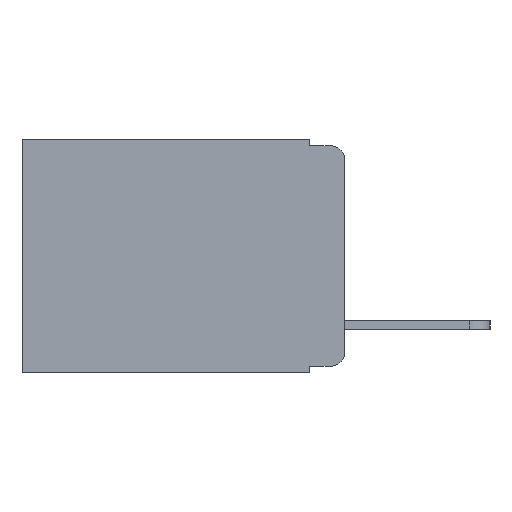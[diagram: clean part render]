
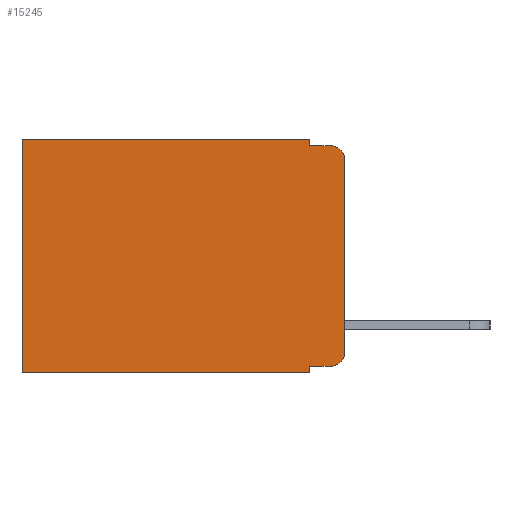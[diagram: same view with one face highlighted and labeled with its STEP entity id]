
A CAD part, left-side view. The second image highlights one B-rep face of the part: STEP entity #15245.
In plain terms, the highlighted planar face has unit normal (-1, 0, 0).
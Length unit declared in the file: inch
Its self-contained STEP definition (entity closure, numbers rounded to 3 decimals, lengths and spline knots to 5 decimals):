
#804 = EDGE_CURVE ( 'NONE', #1659, #19259, #18995, .T. ) ;
#1427 = ORIENTED_EDGE ( 'NONE', *, *, #19930, .F. ) ;
#1541 = VERTEX_POINT ( 'NONE', #19430 ) ;
#1659 = VERTEX_POINT ( 'NONE', #11675 ) ;
#1983 = CARTESIAN_POINT ( 'NONE',  ( 0.298, 0., 0. ) ) ;
#2524 = DIRECTION ( 'NONE',  ( 1., 0., 0. ) ) ;
#2608 = VERTEX_POINT ( 'NONE', #17991 ) ;
#2651 = CARTESIAN_POINT ( 'NONE',  ( 0.298, 0.051, 0. ) ) ;
#3153 = VECTOR ( 'NONE', #8821, 39.37008 ) ;
#3342 = CARTESIAN_POINT ( 'NONE',  ( 0.298, 0.02, -0.03 ) ) ;
#3826 = LINE ( 'NONE', #1983, #6057 ) ;
#3837 = EDGE_LOOP ( 'NONE', ( #9085, #19552, #1427, #15237, #8240, #5613, #4103, #15932, #8895, #5315 ) ) ;
#3910 = EDGE_CURVE ( 'NONE', #18006, #1541, #3826, .T. ) ;
#4018 = VECTOR ( 'NONE', #17475, 39.37008 ) ;
#4103 = ORIENTED_EDGE ( 'NONE', *, *, #4370, .F. ) ;
#4201 = CARTESIAN_POINT ( 'NONE',  ( 0.298, 0.051, -0.333 ) ) ;
#4370 = EDGE_CURVE ( 'NONE', #8781, #20266, #4788, .T. ) ;
#4447 = CARTESIAN_POINT ( 'NONE',  ( 0.298, 0.02, -0.333 ) ) ;
#4701 = FACE_OUTER_BOUND ( 'NONE', #3837, .T. ) ;
#4788 = LINE ( 'NONE', #6445, #17816 ) ;
#5025 = CARTESIAN_POINT ( 'NONE',  ( 0.298, 0.051, 0. ) ) ;
#5315 = ORIENTED_EDGE ( 'NONE', *, *, #8190, .T. ) ;
#5613 = ORIENTED_EDGE ( 'NONE', *, *, #15004, .T. ) ;
#5956 = VECTOR ( 'NONE', #14462, 39.37008 ) ;
#6057 = VECTOR ( 'NONE', #9765, 39.37008 ) ;
#6445 = CARTESIAN_POINT ( 'NONE',  ( 0.298, 0., -0.343 ) ) ;
#6556 = EDGE_CURVE ( 'NONE', #2608, #8781, #13893, .T. ) ;
#6923 = VECTOR ( 'NONE', #17191, 39.37008 ) ;
#7370 = CARTESIAN_POINT ( 'NONE',  ( 0.298, 0.051, -0.01 ) ) ;
#7547 = VERTEX_POINT ( 'NONE', #9221 ) ;
#7624 = DIRECTION ( 'NONE',  ( -1., 0., 0. ) ) ;
#7832 = LINE ( 'NONE', #4201, #3153 ) ;
#7934 = CARTESIAN_POINT ( 'NONE',  ( 0.298, 0.051, -0.01 ) ) ;
#8190 = EDGE_CURVE ( 'NONE', #15485, #1541, #9216, .T. ) ;
#8240 = ORIENTED_EDGE ( 'NONE', *, *, #804, .T. ) ;
#8648 = PLANE ( 'NONE',  #8664 ) ;
#8664 = AXIS2_PLACEMENT_3D ( 'NONE', #11965, #2524, #16770 ) ;
#8781 = VERTEX_POINT ( 'NONE', #13711 ) ;
#8821 = DIRECTION ( 'NONE',  ( 0., -1., 0. ) ) ;
#8895 = ORIENTED_EDGE ( 'NONE', *, *, #17931, .T. ) ;
#8991 = DIRECTION ( 'NONE',  ( 0., 0., -1. ) ) ;
#9085 = ORIENTED_EDGE ( 'NONE', *, *, #3910, .F. ) ;
#9190 = AXIS2_PLACEMENT_3D ( 'NONE', #3342, #14556, #13048 ) ;
#9216 = CIRCLE ( 'NONE', #16793, 0.02 ) ;
#9221 = CARTESIAN_POINT ( 'NONE',  ( 0.298, 0.02, -0.01 ) ) ;
#9341 = DIRECTION ( 'NONE',  ( 0., -1., 0. ) ) ;
#9765 = DIRECTION ( 'NONE',  ( 0., 0., -1. ) ) ;
#9852 = VECTOR ( 'NONE', #8991, 39.37008 ) ;
#10584 = EDGE_CURVE ( 'NONE', #1659, #13709, #18211, .T. ) ;
#10922 = DIRECTION ( 'NONE',  ( 0., 1., 0. ) ) ;
#11094 = VECTOR ( 'NONE', #9341, 39.37008 ) ;
#11675 = CARTESIAN_POINT ( 'NONE',  ( 0.298, 0.051, 0. ) ) ;
#11965 = CARTESIAN_POINT ( 'NONE',  ( 0.298, 0., 0. ) ) ;
#13048 = DIRECTION ( 'NONE',  ( 0., 0., -1. ) ) ;
#13709 = VERTEX_POINT ( 'NONE', #7370 ) ;
#13711 = CARTESIAN_POINT ( 'NONE',  ( 0.298, 0.051, -0.343 ) ) ;
#13893 = LINE ( 'NONE', #5025, #4018 ) ;
#14462 = DIRECTION ( 'NONE',  ( 0., 1., 0. ) ) ;
#14556 = DIRECTION ( 'NONE',  ( -1., 0., 0. ) ) ;
#14774 = LINE ( 'NONE', #7934, #11094 ) ;
#15004 = EDGE_CURVE ( 'NONE', #19259, #20266, #19237, .T. ) ;
#15237 = ORIENTED_EDGE ( 'NONE', *, *, #10584, .F. ) ;
#15245 = ADVANCED_FACE ( 'NONE', ( #4701 ), #8648, .F. ) ;
#15270 = CIRCLE ( 'NONE', #9190, 0.02 ) ;
#15485 = VERTEX_POINT ( 'NONE', #4447 ) ;
#15557 = CARTESIAN_POINT ( 'NONE',  ( 0.298, 0., 0. ) ) ;
#15601 = CARTESIAN_POINT ( 'NONE',  ( 0.298, 0.473, 0. ) ) ;
#15655 = DIRECTION ( 'NONE',  ( 0., 0., -1. ) ) ;
#15704 = EDGE_CURVE ( 'NONE', #18006, #7547, #15270, .T. ) ;
#15932 = ORIENTED_EDGE ( 'NONE', *, *, #6556, .F. ) ;
#16770 = DIRECTION ( 'NONE',  ( 0., 0., -1. ) ) ;
#16793 = AXIS2_PLACEMENT_3D ( 'NONE', #17094, #7624, #15655 ) ;
#17094 = CARTESIAN_POINT ( 'NONE',  ( 0.298, 0.02, -0.313 ) ) ;
#17191 = DIRECTION ( 'NONE',  ( 0., 0., -1. ) ) ;
#17245 = CARTESIAN_POINT ( 'NONE',  ( 0.298, 0.473, 0. ) ) ;
#17475 = DIRECTION ( 'NONE',  ( 0., 0., -1. ) ) ;
#17816 = VECTOR ( 'NONE', #10922, 39.37008 ) ;
#17931 = EDGE_CURVE ( 'NONE', #2608, #15485, #7832, .T. ) ;
#17991 = CARTESIAN_POINT ( 'NONE',  ( 0.298, 0.051, -0.333 ) ) ;
#18006 = VERTEX_POINT ( 'NONE', #18304 ) ;
#18086 = CARTESIAN_POINT ( 'NONE',  ( 0.298, 0.473, -0.343 ) ) ;
#18211 = LINE ( 'NONE', #2651, #9852 ) ;
#18304 = CARTESIAN_POINT ( 'NONE',  ( 0.298, 0., -0.03 ) ) ;
#18995 = LINE ( 'NONE', #15557, #5956 ) ;
#19237 = LINE ( 'NONE', #15601, #6923 ) ;
#19259 = VERTEX_POINT ( 'NONE', #17245 ) ;
#19430 = CARTESIAN_POINT ( 'NONE',  ( 0.298, 0., -0.313 ) ) ;
#19552 = ORIENTED_EDGE ( 'NONE', *, *, #15704, .T. ) ;
#19930 = EDGE_CURVE ( 'NONE', #13709, #7547, #14774, .T. ) ;
#20266 = VERTEX_POINT ( 'NONE', #18086 ) ;
